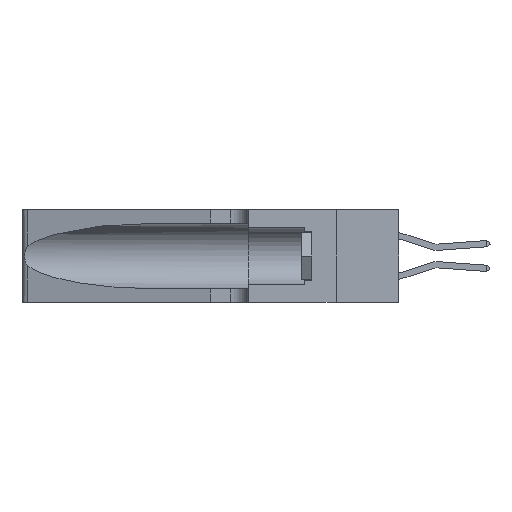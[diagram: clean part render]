
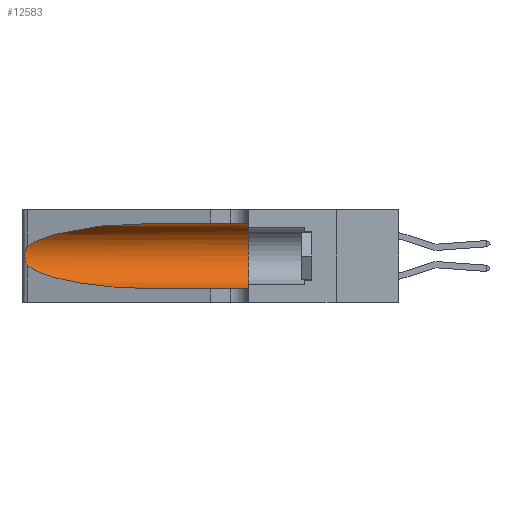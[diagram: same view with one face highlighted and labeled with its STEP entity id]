
A CAD part, left-side view. The second image highlights one B-rep face of the part: STEP entity #12583.
In plain terms, the highlighted cylindrical face has radius 3.308 mm (diameter 6.617 mm), a partial arc.
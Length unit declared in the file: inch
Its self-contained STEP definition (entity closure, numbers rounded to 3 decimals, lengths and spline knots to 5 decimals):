
#79 = CARTESIAN_POINT ( 'NONE',  ( 0.1305, 1.61858, 0.185 ) ) ;
#413 = CARTESIAN_POINT ( 'NONE',  ( 0.25787, 1.23484, 0.2124 ) ) ;
#1058 = VERTEX_POINT ( 'NONE', #12703 ) ;
#1323 = DIRECTION ( 'NONE',  ( 0., 1., 0. ) ) ;
#2051 = CARTESIAN_POINT ( 'NONE',  ( 0.26018, 1.23835, 0.19895 ) ) ;
#2084 = CIRCLE ( 'NONE', #20346, 0.13025 ) ;
#2964 = ORIENTED_EDGE ( 'NONE', *, *, #21304, .F. ) ;
#3588 = CARTESIAN_POINT ( 'NONE',  ( 0.1305, 1.61858, 0.31525 ) ) ;
#3698 = CARTESIAN_POINT ( 'NONE',  ( 0.26075, 1.23896, 0.178 ) ) ;
#3980 = EDGE_LOOP ( 'NONE', ( #14095, #20723, #21188, #19614, #2964, #5080 ) ) ;
#4336 = CARTESIAN_POINT ( 'NONE',  ( 0.1305, 0.35, 0.05475 ) ) ;
#4792 = LINE ( 'NONE', #3588, #18108 ) ;
#4921 = CARTESIAN_POINT ( 'NONE',  ( 0.25487, 1.22718, 0.22369 ) ) ;
#5080 = ORIENTED_EDGE ( 'NONE', *, *, #9161, .F. ) ;
#5282 = DIRECTION ( 'NONE',  ( 0., -1., 0. ) ) ;
#5386 = CARTESIAN_POINT ( 'NONE',  ( 0.25856, 1.23593, 0.16098 ) ) ;
#5663 = CARTESIAN_POINT ( 'NONE',  ( 0.25487, 1.22718, 0.14631 ) ) ;
#6994 = CARTESIAN_POINT ( 'NONE',  ( 0.25555, 1.22994, 0.2215 ) ) ;
#7069 = CARTESIAN_POINT ( 'NONE',  ( 0.25639, 1.23186, 0.15144 ) ) ;
#7336 = CARTESIAN_POINT ( 'NONE',  ( 0.1305, 0.72297, 0.05475 ) ) ;
#8714 = CARTESIAN_POINT ( 'NONE',  ( 0.25487, 1.22718, 0.14631 ) ) ;
#8786 = VERTEX_POINT ( 'NONE', #10381 ) ;
#9161 = EDGE_CURVE ( 'NONE', #8786, #10753, #4792, .T. ) ;
#9613 =( BOUNDED_CURVE ( )  B_SPLINE_CURVE ( 3, ( #5663, #15667, #17332, #7336 ),
 .UNSPECIFIED., .F., .T. ) 
 B_SPLINE_CURVE_WITH_KNOTS ( ( 4, 4 ),
 ( 3.44316, 4.71239 ),
 .UNSPECIFIED. ) 
 CURVE ( )  GEOMETRIC_REPRESENTATION_ITEM ( )  RATIONAL_B_SPLINE_CURVE ( ( 1., 0.87, 0.87, 1. ) ) 
 REPRESENTATION_ITEM ( '' )  );
#9781 = CARTESIAN_POINT ( 'NONE',  ( 0.25487, 1.22718, 0.22369 ) ) ;
#10364 = CARTESIAN_POINT ( 'NONE',  ( 0.25639, 1.23184, 0.21858 ) ) ;
#10381 = CARTESIAN_POINT ( 'NONE',  ( 0.1305, 0.72297, 0.31525 ) ) ;
#10753 = VERTEX_POINT ( 'NONE', #11021 ) ;
#10924 = CARTESIAN_POINT ( 'NONE',  ( 0.1305, 1.61858, 0.05475 ) ) ;
#11021 = CARTESIAN_POINT ( 'NONE',  ( 0.1305, 0.35, 0.31525 ) ) ;
#11321 = CARTESIAN_POINT ( 'NONE',  ( 0.1305, 0.35, 0.185 ) ) ;
#11596 = AXIS2_PLACEMENT_3D ( 'NONE', #79, #11741, #18337 ) ;
#11741 = DIRECTION ( 'NONE',  ( 0., -1., 0. ) ) ;
#11939 =( BOUNDED_CURVE ( )  B_SPLINE_CURVE ( 3, ( #19874, #21558, #14924, #4921 ),
 .UNSPECIFIED., .F., .T. ) 
 B_SPLINE_CURVE_WITH_KNOTS ( ( 4, 4 ),
 ( 1.5708, 2.84003 ),
 .UNSPECIFIED. ) 
 CURVE ( )  GEOMETRIC_REPRESENTATION_ITEM ( )  RATIONAL_B_SPLINE_CURVE ( ( 1., 0.87, 0.87, 1. ) ) 
 REPRESENTATION_ITEM ( '' )  );
#12030 = FACE_OUTER_BOUND ( 'NONE', #3980, .T. ) ;
#12072 = CARTESIAN_POINT ( 'NONE',  ( 0.25854, 1.2359, 0.20912 ) ) ;
#12413 = EDGE_CURVE ( 'NONE', #14467, #15865, #16175, .T. ) ;
#12583 = ADVANCED_FACE ( 'NONE', ( #12030 ), #20340, .F. ) ;
#12615 = DIRECTION ( 'NONE',  ( 0., -1., 0. ) ) ;
#12703 = CARTESIAN_POINT ( 'NONE',  ( 0.25487, 1.22718, 0.14631 ) ) ;
#12986 = DIRECTION ( 'NONE',  ( 0., 0., 1. ) ) ;
#13357 = EDGE_CURVE ( 'NONE', #14430, #1058, #17398, .T. ) ;
#13718 = CARTESIAN_POINT ( 'NONE',  ( 0.26075, 1.23896, 0.19203 ) ) ;
#14095 = ORIENTED_EDGE ( 'NONE', *, *, #19667, .T. ) ;
#14116 = EDGE_CURVE ( 'NONE', #1058, #14467, #9613, .T. ) ;
#14430 = VERTEX_POINT ( 'NONE', #9781 ) ;
#14467 = VERTEX_POINT ( 'NONE', #18182 ) ;
#14924 = CARTESIAN_POINT ( 'NONE',  ( 0.2373, 1.15595, 0.28018 ) ) ;
#15393 = CARTESIAN_POINT ( 'NONE',  ( 0.26017, 1.23833, 0.17102 ) ) ;
#15665 = VECTOR ( 'NONE', #12615, 39.37008 ) ;
#15667 = CARTESIAN_POINT ( 'NONE',  ( 0.2373, 1.15595, 0.08982 ) ) ;
#15865 = VERTEX_POINT ( 'NONE', #4336 ) ;
#16175 = LINE ( 'NONE', #10924, #15665 ) ;
#17074 = CARTESIAN_POINT ( 'NONE',  ( 0.25789, 1.23486, 0.15765 ) ) ;
#17332 = CARTESIAN_POINT ( 'NONE',  ( 0.18966, 0.96281, 0.05475 ) ) ;
#17398 = B_SPLINE_CURVE_WITH_KNOTS ( 'NONE', 3,
 ( #18669, #6994, #10364, #413, #12072, #2051, #13718, #3698, #15393, #5386, #17074, #7069, #18749, #8714 ),
 .UNSPECIFIED., .F., .F.,
 ( 4, 2, 2, 2, 2, 2, 4 ),
 ( 0., 0.00027, 0.00053, 0.00107, 0.0016, 0.00187, 0.00214 ),
 .UNSPECIFIED. ) ;
#18108 = VECTOR ( 'NONE', #5282, 39.37008 ) ;
#18182 = CARTESIAN_POINT ( 'NONE',  ( 0.1305, 0.72297, 0.05475 ) ) ;
#18337 = DIRECTION ( 'NONE',  ( 0., 0., -1. ) ) ;
#18669 = CARTESIAN_POINT ( 'NONE',  ( 0.25487, 1.22718, 0.22369 ) ) ;
#18749 = CARTESIAN_POINT ( 'NONE',  ( 0.25555, 1.22993, 0.14849 ) ) ;
#19614 = ORIENTED_EDGE ( 'NONE', *, *, #12413, .T. ) ;
#19667 = EDGE_CURVE ( 'NONE', #8786, #14430, #11939, .T. ) ;
#19874 = CARTESIAN_POINT ( 'NONE',  ( 0.1305, 0.72297, 0.31525 ) ) ;
#20340 = CYLINDRICAL_SURFACE ( 'NONE', #11596, 0.13025 ) ;
#20346 = AXIS2_PLACEMENT_3D ( 'NONE', #11321, #1323, #12986 ) ;
#20723 = ORIENTED_EDGE ( 'NONE', *, *, #13357, .T. ) ;
#21188 = ORIENTED_EDGE ( 'NONE', *, *, #14116, .T. ) ;
#21304 = EDGE_CURVE ( 'NONE', #10753, #15865, #2084, .T. ) ;
#21558 = CARTESIAN_POINT ( 'NONE',  ( 0.18966, 0.96281, 0.31525 ) ) ;
